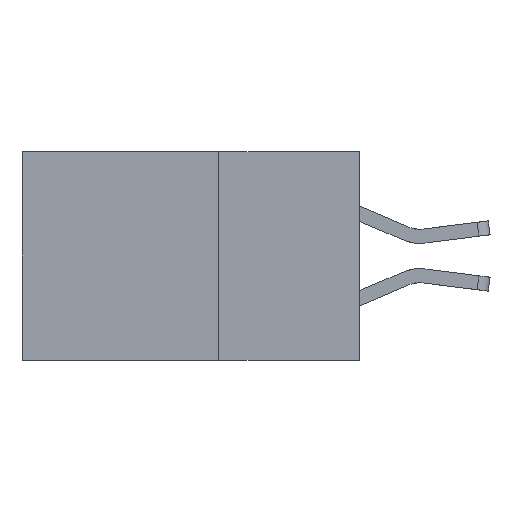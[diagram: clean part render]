
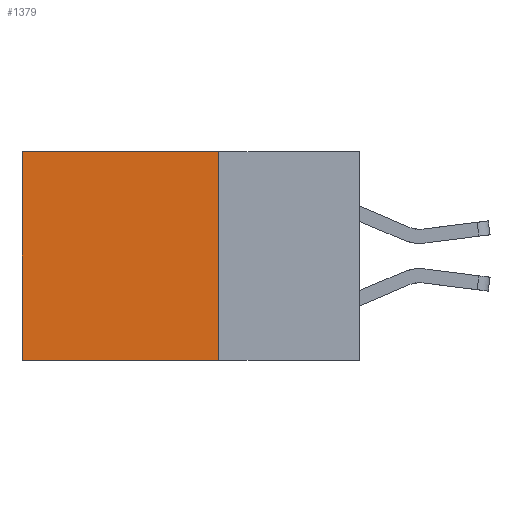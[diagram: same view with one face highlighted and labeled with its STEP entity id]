
A CAD part, left-side view. The second image highlights one B-rep face of the part: STEP entity #1379.
In plain terms, the highlighted planar face has unit normal (-1, 0, 0).
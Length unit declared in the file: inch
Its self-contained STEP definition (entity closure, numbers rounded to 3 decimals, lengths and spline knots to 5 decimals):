
#106 = CARTESIAN_POINT ( 'NONE',  ( 0.2875, 0.6, 0. ) ) ;
#131 = CARTESIAN_POINT ( 'NONE',  ( 0.2875, 0.6, 0. ) ) ;
#944 = EDGE_CURVE ( 'NONE', #5184, #4872, #10417, .T. ) ;
#1379 = ADVANCED_FACE ( 'NONE', ( #1981 ), #8951, .F. ) ;
#1742 = DIRECTION ( 'NONE',  ( 0., 0., -1. ) ) ;
#1981 = FACE_OUTER_BOUND ( 'NONE', #9247, .T. ) ;
#3144 = LINE ( 'NONE', #3542, #5430 ) ;
#3362 = CARTESIAN_POINT ( 'NONE',  ( 0.2875, 0.25, 0. ) ) ;
#3489 = CARTESIAN_POINT ( 'NONE',  ( 0.2875, 0.25, 0. ) ) ;
#3542 = CARTESIAN_POINT ( 'NONE',  ( 0.2875, 0.25, -0.37 ) ) ;
#4320 = ORIENTED_EDGE ( 'NONE', *, *, #944, .T. ) ;
#4347 = ORIENTED_EDGE ( 'NONE', *, *, #10323, .T. ) ;
#4559 = DIRECTION ( 'NONE',  ( 1., 0., 0. ) ) ;
#4727 = VERTEX_POINT ( 'NONE', #7309 ) ;
#4852 = VECTOR ( 'NONE', #8392, 39.37008 ) ;
#4872 = VERTEX_POINT ( 'NONE', #5035 ) ;
#5035 = CARTESIAN_POINT ( 'NONE',  ( 0.2875, 0.6, -0.37 ) ) ;
#5075 = EDGE_CURVE ( 'NONE', #6701, #4727, #6887, .T. ) ;
#5184 = VERTEX_POINT ( 'NONE', #131 ) ;
#5205 = CARTESIAN_POINT ( 'NONE',  ( 0.2875, 0.25, 0. ) ) ;
#5430 = VECTOR ( 'NONE', #9374, 39.37008 ) ;
#6701 = VERTEX_POINT ( 'NONE', #5205 ) ;
#6723 = EDGE_CURVE ( 'NONE', #4727, #4872, #3144, .T. ) ;
#6887 = LINE ( 'NONE', #11042, #9085 ) ;
#6923 = ORIENTED_EDGE ( 'NONE', *, *, #6723, .F. ) ;
#7309 = CARTESIAN_POINT ( 'NONE',  ( 0.2875, 0.25, -0.37 ) ) ;
#7773 = DIRECTION ( 'NONE',  ( 0., 0., -1. ) ) ;
#8392 = DIRECTION ( 'NONE',  ( 0., 1., 0. ) ) ;
#8499 = VECTOR ( 'NONE', #11031, 39.37008 ) ;
#8951 = PLANE ( 'NONE',  #9960 ) ;
#9085 = VECTOR ( 'NONE', #7773, 39.37008 ) ;
#9228 = LINE ( 'NONE', #3362, #4852 ) ;
#9247 = EDGE_LOOP ( 'NONE', ( #4320, #6923, #10187, #4347 ) ) ;
#9374 = DIRECTION ( 'NONE',  ( 0., 1., 0. ) ) ;
#9960 = AXIS2_PLACEMENT_3D ( 'NONE', #3489, #4559, #1742 ) ;
#10187 = ORIENTED_EDGE ( 'NONE', *, *, #5075, .F. ) ;
#10323 = EDGE_CURVE ( 'NONE', #6701, #5184, #9228, .T. ) ;
#10417 = LINE ( 'NONE', #106, #8499 ) ;
#11031 = DIRECTION ( 'NONE',  ( 0., 0., -1. ) ) ;
#11042 = CARTESIAN_POINT ( 'NONE',  ( 0.2875, 0.25, 0. ) ) ;
